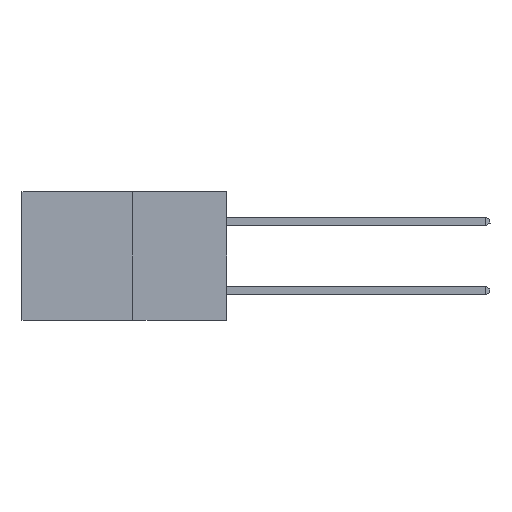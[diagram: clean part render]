
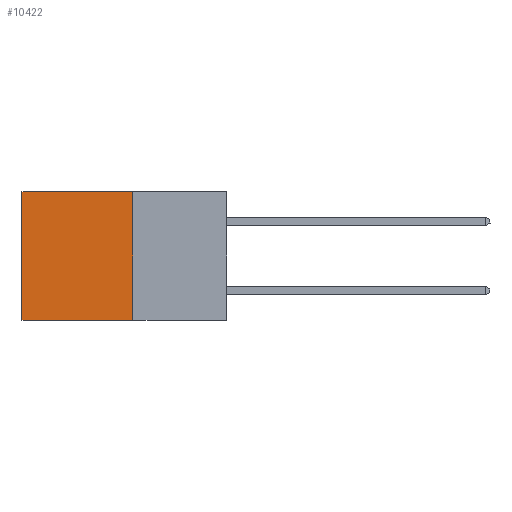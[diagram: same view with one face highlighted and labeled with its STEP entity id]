
A CAD part, left-side view. The second image highlights one B-rep face of the part: STEP entity #10422.
In plain terms, the highlighted planar face has unit normal (-1, 0, 0).
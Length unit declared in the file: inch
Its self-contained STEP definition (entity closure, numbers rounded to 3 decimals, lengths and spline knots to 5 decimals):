
#257 = LINE ( 'NONE', #7810, #10731 ) ;
#312 = DIRECTION ( 'NONE',  ( 0., 0., -1. ) ) ;
#337 = ORIENTED_EDGE ( 'NONE', *, *, #455, .F. ) ;
#455 = EDGE_CURVE ( 'NONE', #5921, #5993, #257, .T. ) ;
#730 = ORIENTED_EDGE ( 'NONE', *, *, #3945, .T. ) ;
#900 = CARTESIAN_POINT ( 'NONE',  ( 0.277, 0.27, -0.37 ) ) ;
#1073 = FACE_OUTER_BOUND ( 'NONE', #1933, .T. ) ;
#1106 = PLANE ( 'NONE',  #9773 ) ;
#1933 = EDGE_LOOP ( 'NONE', ( #730, #337, #4603, #9643 ) ) ;
#2398 = CARTESIAN_POINT ( 'NONE',  ( 0.277, 0.59, -0.37 ) ) ;
#3146 = DIRECTION ( 'NONE',  ( 1., 0., 0. ) ) ;
#3945 = EDGE_CURVE ( 'NONE', #10058, #5993, #9416, .T. ) ;
#4264 = CARTESIAN_POINT ( 'NONE',  ( 0.277, 0.27, -0.37 ) ) ;
#4603 = ORIENTED_EDGE ( 'NONE', *, *, #12126, .F. ) ;
#5044 = CARTESIAN_POINT ( 'NONE',  ( 0.277, 0.59, -0.37 ) ) ;
#5921 = VERTEX_POINT ( 'NONE', #900 ) ;
#5993 = VERTEX_POINT ( 'NONE', #5044 ) ;
#6905 = VECTOR ( 'NONE', #312, 39.37008 ) ;
#7202 = DIRECTION ( 'NONE',  ( 0., 0., -1. ) ) ;
#7810 = CARTESIAN_POINT ( 'NONE',  ( 0.277, 0.27, -0.37 ) ) ;
#8007 = VECTOR ( 'NONE', #11163, 39.37008 ) ;
#8604 = VERTEX_POINT ( 'NONE', #11350 ) ;
#8962 = CARTESIAN_POINT ( 'NONE',  ( 0.277, 0.27, -0.37 ) ) ;
#9181 = VECTOR ( 'NONE', #7202, 39.37008 ) ;
#9416 = LINE ( 'NONE', #2398, #6905 ) ;
#9643 = ORIENTED_EDGE ( 'NONE', *, *, #12248, .T. ) ;
#9773 = AXIS2_PLACEMENT_3D ( 'NONE', #8962, #3146, #9938 ) ;
#9938 = DIRECTION ( 'NONE',  ( 0., 0., -1. ) ) ;
#10058 = VERTEX_POINT ( 'NONE', #10439 ) ;
#10161 = CARTESIAN_POINT ( 'NONE',  ( 0.277, 0.27, 0. ) ) ;
#10422 = ADVANCED_FACE ( 'NONE', ( #1073 ), #1106, .F. ) ;
#10439 = CARTESIAN_POINT ( 'NONE',  ( 0.277, 0.59, 0. ) ) ;
#10731 = VECTOR ( 'NONE', #11703, 39.37008 ) ;
#11137 = LINE ( 'NONE', #10161, #8007 ) ;
#11163 = DIRECTION ( 'NONE',  ( 0., 1., 0. ) ) ;
#11350 = CARTESIAN_POINT ( 'NONE',  ( 0.277, 0.27, 0. ) ) ;
#11703 = DIRECTION ( 'NONE',  ( 0., 1., 0. ) ) ;
#12043 = LINE ( 'NONE', #4264, #9181 ) ;
#12126 = EDGE_CURVE ( 'NONE', #8604, #5921, #12043, .T. ) ;
#12248 = EDGE_CURVE ( 'NONE', #8604, #10058, #11137, .T. ) ;
